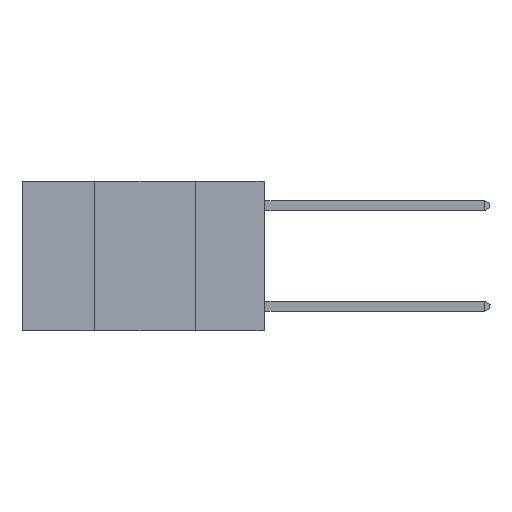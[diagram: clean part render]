
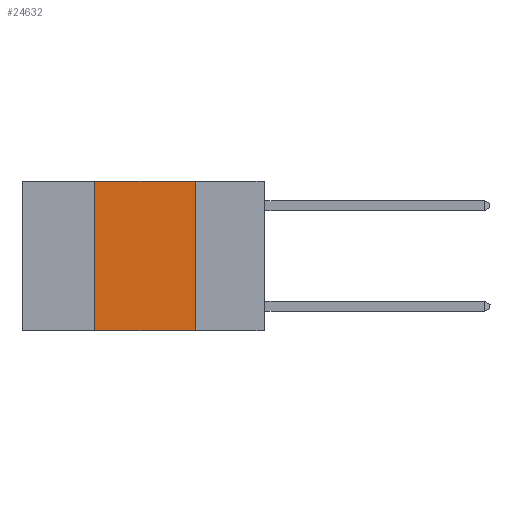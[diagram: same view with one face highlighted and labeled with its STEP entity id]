
A CAD part, left-side view. The second image highlights one B-rep face of the part: STEP entity #24632.
In plain terms, the highlighted planar face has unit normal (-1, 0, 0).
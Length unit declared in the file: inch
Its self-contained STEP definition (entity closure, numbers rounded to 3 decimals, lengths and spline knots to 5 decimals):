
#176 = CARTESIAN_POINT ( 'NONE',  ( 0., 0.6, 0. ) ) ;
#475 = LINE ( 'NONE', #5040, #22608 ) ;
#740 = VERTEX_POINT ( 'NONE', #4014 ) ;
#2350 = DIRECTION ( 'NONE',  ( 1., 0., 0. ) ) ;
#3281 = AXIS2_PLACEMENT_3D ( 'NONE', #176, #2350, #17379 ) ;
#4014 = CARTESIAN_POINT ( 'NONE',  ( 0., 0.42, -0.37 ) ) ;
#4554 = EDGE_CURVE ( 'NONE', #6521, #27013, #475, .T. ) ;
#5040 = CARTESIAN_POINT ( 'NONE',  ( 0., 0.17, 0. ) ) ;
#5072 = ORIENTED_EDGE ( 'NONE', *, *, #16030, .T. ) ;
#6298 = CARTESIAN_POINT ( 'NONE',  ( 0., 0.42, 0. ) ) ;
#6521 = VERTEX_POINT ( 'NONE', #16983 ) ;
#7509 = CARTESIAN_POINT ( 'NONE',  ( 0., 0.17, -0.37 ) ) ;
#7789 = LINE ( 'NONE', #14016, #13415 ) ;
#8813 = ORIENTED_EDGE ( 'NONE', *, *, #4554, .F. ) ;
#9242 = VECTOR ( 'NONE', #24796, 39.37008 ) ;
#9407 = DIRECTION ( 'NONE',  ( 0., 0., -1. ) ) ;
#10129 = ORIENTED_EDGE ( 'NONE', *, *, #12106, .F. ) ;
#11402 = EDGE_LOOP ( 'NONE', ( #8813, #10129, #15782, #5072 ) ) ;
#11764 = EDGE_CURVE ( 'NONE', #740, #18487, #13554, .T. ) ;
#12106 = EDGE_CURVE ( 'NONE', #18487, #6521, #20600, .T. ) ;
#13035 = PLANE ( 'NONE',  #3281 ) ;
#13415 = VECTOR ( 'NONE', #18349, 39.37008 ) ;
#13554 = LINE ( 'NONE', #23673, #18594 ) ;
#14016 = CARTESIAN_POINT ( 'NONE',  ( 0., 0.6, -0.37 ) ) ;
#15782 = ORIENTED_EDGE ( 'NONE', *, *, #11764, .F. ) ;
#16030 = EDGE_CURVE ( 'NONE', #740, #27013, #7789, .T. ) ;
#16173 = CARTESIAN_POINT ( 'NONE',  ( 0., 0.6, 0. ) ) ;
#16983 = CARTESIAN_POINT ( 'NONE',  ( 0., 0.17, 0. ) ) ;
#17379 = DIRECTION ( 'NONE',  ( 0., 0., -1. ) ) ;
#18349 = DIRECTION ( 'NONE',  ( 0., -1., 0. ) ) ;
#18487 = VERTEX_POINT ( 'NONE', #6298 ) ;
#18594 = VECTOR ( 'NONE', #21538, 39.37008 ) ;
#20600 = LINE ( 'NONE', #16173, #9242 ) ;
#21329 = FACE_OUTER_BOUND ( 'NONE', #11402, .T. ) ;
#21538 = DIRECTION ( 'NONE',  ( 0., 0., 1. ) ) ;
#22608 = VECTOR ( 'NONE', #9407, 39.37008 ) ;
#23673 = CARTESIAN_POINT ( 'NONE',  ( 0., 0.42, 0. ) ) ;
#24632 = ADVANCED_FACE ( 'NONE', ( #21329 ), #13035, .F. ) ;
#24796 = DIRECTION ( 'NONE',  ( 0., -1., 0. ) ) ;
#27013 = VERTEX_POINT ( 'NONE', #7509 ) ;
